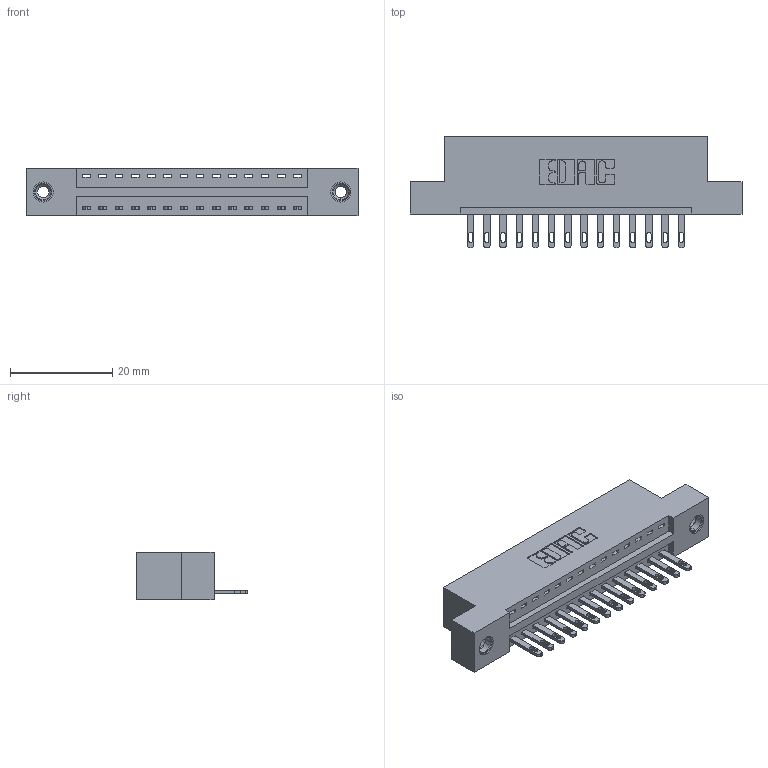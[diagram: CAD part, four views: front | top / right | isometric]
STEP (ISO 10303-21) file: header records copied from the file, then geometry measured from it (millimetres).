
FILE_DESCRIPTION (( 'STEP AP203' ), '1' );
FILE_NAME ('896-014-500-108.STEP', '2021-07-27T15:10:03', ( '' ), ( '' ), 'SwSTEP 2.0', 'SolidWorks 2020', '' );
FILE_SCHEMA (( 'CONFIG_CONTROL_DESIGN' ));
Length unit declared in the file: inch
Products named in the file (4): 846 Part_Flush Mounting Lugs - 0.156 Dia-TI; 896-014-500-108; 345-292-001_345-293-100; 345-250-001_345-250-003-102
Assembly tree (17 placements, depth 2):
  896-014-500-108
    846 Part_Flush Mounting Lugs - 0.156 Dia-TI
    345-292-001_345-293-100  x14
    345-250-001_345-250-003-102  x2
Bounding box: 65.02 x 21.84 x 9.4 mm (x, y, z)
Volume: 6033.5 mm3; surface area: 7293.3 mm2
Topology: 17 solids, 17 shells, 938 faces, 2817 edges, 1870 vertices
Faces by surface type: plane 584, cylinder 338, cone 12, torus 4
Entity records: 13574 total; most frequent: CARTESIAN_POINT 2317, ORIENTED_EDGE 2258, DIRECTION 2107, EDGE_CURVE 1129, LINE 917, VECTOR 917, VERTEX_POINT 748, AXIS2_PLACEMENT_3D 595
